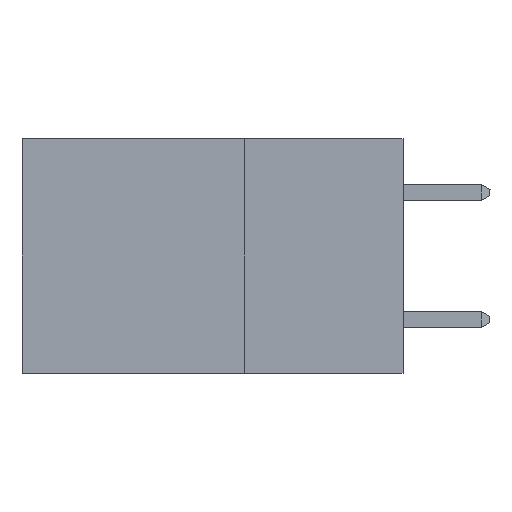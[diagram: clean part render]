
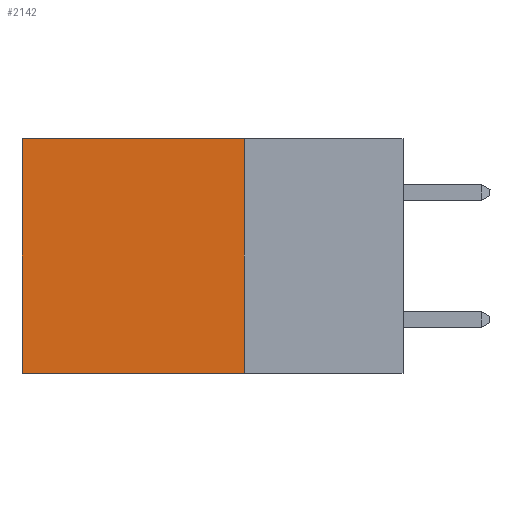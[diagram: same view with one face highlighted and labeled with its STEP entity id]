
A CAD part, left-side view. The second image highlights one B-rep face of the part: STEP entity #2142.
In plain terms, the highlighted planar face has unit normal (-1, 0, 0).
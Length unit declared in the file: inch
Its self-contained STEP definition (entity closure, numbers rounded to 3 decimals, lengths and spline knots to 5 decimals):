
#469 = VECTOR ( 'NONE', #1444, 39.37008 ) ;
#840 = VERTEX_POINT ( 'NONE', #4434 ) ;
#916 = DIRECTION ( 'NONE',  ( 0., 0., -1. ) ) ;
#1051 = EDGE_CURVE ( 'NONE', #840, #7332, #1786, .T. ) ;
#1186 = VECTOR ( 'NONE', #10442, 39.37008 ) ;
#1231 = EDGE_CURVE ( 'NONE', #8581, #1495, #2315, .T. ) ;
#1444 = DIRECTION ( 'NONE',  ( 0., 1., 0. ) ) ;
#1495 = VERTEX_POINT ( 'NONE', #8643 ) ;
#1786 = LINE ( 'NONE', #5001, #9409 ) ;
#2142 = ADVANCED_FACE ( 'NONE', ( #5389 ), #7662, .F. ) ;
#2315 = LINE ( 'NONE', #6392, #469 ) ;
#2523 = EDGE_CURVE ( 'NONE', #7332, #1495, #6195, .T. ) ;
#3625 = ORIENTED_EDGE ( 'NONE', *, *, #1231, .F. ) ;
#3629 = DIRECTION ( 'NONE',  ( 0., 0., -1. ) ) ;
#3630 = CARTESIAN_POINT ( 'NONE',  ( 0.2875, 0.25, 0. ) ) ;
#4140 = DIRECTION ( 'NONE',  ( 0., 1., 0. ) ) ;
#4197 = CARTESIAN_POINT ( 'NONE',  ( 0.2875, 0.25, 0. ) ) ;
#4378 = CARTESIAN_POINT ( 'NONE',  ( 0.2875, 0.6, 0. ) ) ;
#4434 = CARTESIAN_POINT ( 'NONE',  ( 0.2875, 0.25, 0. ) ) ;
#4545 = EDGE_LOOP ( 'NONE', ( #4619, #3625, #8717, #9703 ) ) ;
#4576 = EDGE_CURVE ( 'NONE', #840, #8581, #6452, .T. ) ;
#4619 = ORIENTED_EDGE ( 'NONE', *, *, #2523, .T. ) ;
#5001 = CARTESIAN_POINT ( 'NONE',  ( 0.2875, 0.25, 0. ) ) ;
#5389 = FACE_OUTER_BOUND ( 'NONE', #4545, .T. ) ;
#5502 = CARTESIAN_POINT ( 'NONE',  ( 0.2875, 0.25, -0.37 ) ) ;
#5525 = AXIS2_PLACEMENT_3D ( 'NONE', #4197, #5932, #916 ) ;
#5932 = DIRECTION ( 'NONE',  ( 1., 0., 0. ) ) ;
#6195 = LINE ( 'NONE', #4378, #9914 ) ;
#6392 = CARTESIAN_POINT ( 'NONE',  ( 0.2875, 0.25, -0.37 ) ) ;
#6452 = LINE ( 'NONE', #3630, #1186 ) ;
#7332 = VERTEX_POINT ( 'NONE', #8843 ) ;
#7662 = PLANE ( 'NONE',  #5525 ) ;
#8581 = VERTEX_POINT ( 'NONE', #5502 ) ;
#8643 = CARTESIAN_POINT ( 'NONE',  ( 0.2875, 0.6, -0.37 ) ) ;
#8717 = ORIENTED_EDGE ( 'NONE', *, *, #4576, .F. ) ;
#8843 = CARTESIAN_POINT ( 'NONE',  ( 0.2875, 0.6, 0. ) ) ;
#9409 = VECTOR ( 'NONE', #4140, 39.37008 ) ;
#9703 = ORIENTED_EDGE ( 'NONE', *, *, #1051, .T. ) ;
#9914 = VECTOR ( 'NONE', #3629, 39.37008 ) ;
#10442 = DIRECTION ( 'NONE',  ( 0., 0., -1. ) ) ;
